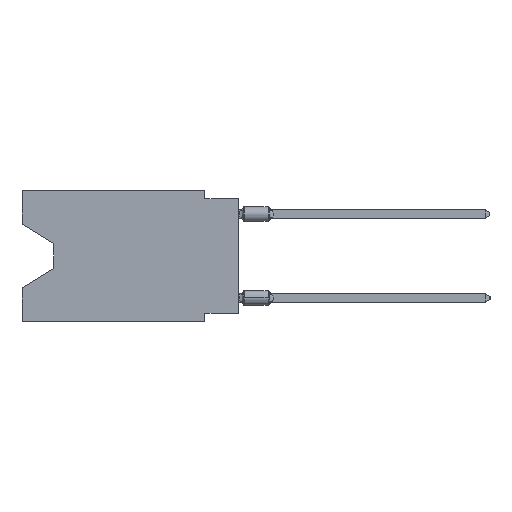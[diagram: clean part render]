
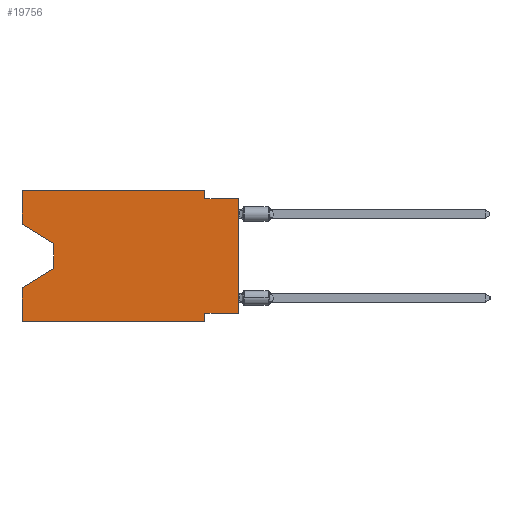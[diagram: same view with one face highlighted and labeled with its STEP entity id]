
A CAD part, left-side view. The second image highlights one B-rep face of the part: STEP entity #19756.
In plain terms, the highlighted planar face has unit normal (-1, 0, 0).
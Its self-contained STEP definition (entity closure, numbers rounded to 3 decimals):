
#735 = EDGE_CURVE ( 'NONE', #19080, #23410, #14116, .T. ) ;
#750 = EDGE_CURVE ( 'NONE', #18447, #24521, #22341, .T. ) ;
#1226 = VERTEX_POINT ( 'NONE', #35129 ) ;
#1673 = CARTESIAN_POINT ( 'NONE',  ( 0., 2.54, -9.906 ) ) ;
#1830 = ORIENTED_EDGE ( 'NONE', *, *, #34242, .T. ) ;
#2940 = LINE ( 'NONE', #16898, #18872 ) ;
#3154 = CARTESIAN_POINT ( 'NONE',  ( 0., 0., 0. ) ) ;
#3334 = VERTEX_POINT ( 'NONE', #30031 ) ;
#3499 = DIRECTION ( 'NONE',  ( 0., 0., 1. ) ) ;
#3804 = VECTOR ( 'NONE', #29965, 1000. ) ;
#3872 = EDGE_CURVE ( 'NONE', #23806, #32056, #2940, .T. ) ;
#4715 = VECTOR ( 'NONE', #9165, 1000. ) ;
#5166 = DIRECTION ( 'NONE',  ( 1., 0., 0. ) ) ;
#5178 = LINE ( 'NONE', #22177, #27597 ) ;
#5519 = VECTOR ( 'NONE', #27559, 1000. ) ;
#5524 = PLANE ( 'NONE',  #31089 ) ;
#5716 = CARTESIAN_POINT ( 'NONE',  ( 0., 13.97, -5.893 ) ) ;
#5723 = LINE ( 'NONE', #16637, #5519 ) ;
#6647 = CARTESIAN_POINT ( 'NONE',  ( 0., 16.383, 0. ) ) ;
#7256 = VERTEX_POINT ( 'NONE', #1673 ) ;
#7344 = ORIENTED_EDGE ( 'NONE', *, *, #23387, .T. ) ;
#7484 = DIRECTION ( 'NONE',  ( 0., 0., 1. ) ) ;
#7715 = ORIENTED_EDGE ( 'NONE', *, *, #8656, .T. ) ;
#8090 = ORIENTED_EDGE ( 'NONE', *, *, #29186, .F. ) ;
#8298 = LINE ( 'NONE', #16544, #3804 ) ;
#8651 = DIRECTION ( 'NONE',  ( 0., 0.855, -0.519 ) ) ;
#8656 = EDGE_CURVE ( 'NONE', #31362, #3334, #27870, .T. ) ;
#9117 = VECTOR ( 'NONE', #14319, 1000. ) ;
#9165 = DIRECTION ( 'NONE',  ( 0., 0., -1. ) ) ;
#9995 = ORIENTED_EDGE ( 'NONE', *, *, #19413, .F. ) ;
#10466 = LINE ( 'NONE', #21583, #16345 ) ;
#11250 = FACE_OUTER_BOUND ( 'NONE', #31777, .T. ) ;
#11430 = DIRECTION ( 'NONE',  ( 0., -1., 0. ) ) ;
#12845 = CARTESIAN_POINT ( 'NONE',  ( 0., 16.383, 0. ) ) ;
#13225 = LINE ( 'NONE', #26847, #4715 ) ;
#13227 = VECTOR ( 'NONE', #33432, 1000. ) ;
#13582 = CARTESIAN_POINT ( 'NONE',  ( 0., 16.383, 0. ) ) ;
#13848 = EDGE_CURVE ( 'NONE', #23806, #7256, #8298, .T. ) ;
#14116 = LINE ( 'NONE', #30246, #22377 ) ;
#14216 = VERTEX_POINT ( 'NONE', #5716 ) ;
#14256 = ORIENTED_EDGE ( 'NONE', *, *, #34443, .F. ) ;
#14319 = DIRECTION ( 'NONE',  ( 0., 0., -1. ) ) ;
#15009 = CARTESIAN_POINT ( 'NONE',  ( 0., 2.54, -9.906 ) ) ;
#15659 = ORIENTED_EDGE ( 'NONE', *, *, #3872, .F. ) ;
#15856 = DIRECTION ( 'NONE',  ( 0., 1., 0. ) ) ;
#16086 = DIRECTION ( 'NONE',  ( 0., 0., -1. ) ) ;
#16345 = VECTOR ( 'NONE', #15856, 1000. ) ;
#16544 = CARTESIAN_POINT ( 'NONE',  ( 0., 16.383, -9.906 ) ) ;
#16637 = CARTESIAN_POINT ( 'NONE',  ( 0., 0., -0.635 ) ) ;
#16898 = CARTESIAN_POINT ( 'NONE',  ( 0., 16.383, 0. ) ) ;
#18447 = VERTEX_POINT ( 'NONE', #23692 ) ;
#18872 = VECTOR ( 'NONE', #19949, 1000. ) ;
#19080 = VERTEX_POINT ( 'NONE', #6647 ) ;
#19363 = VECTOR ( 'NONE', #3499, 1000. ) ;
#19413 = EDGE_CURVE ( 'NONE', #1226, #7256, #30805, .T. ) ;
#19756 = ADVANCED_FACE ( 'NONE', ( #11250 ), #5524, .F. ) ;
#19949 = DIRECTION ( 'NONE',  ( 0., 0., 1. ) ) ;
#21260 = EDGE_CURVE ( 'NONE', #18447, #19080, #31859, .T. ) ;
#21583 = CARTESIAN_POINT ( 'NONE',  ( 0., 0., -9.271 ) ) ;
#22177 = CARTESIAN_POINT ( 'NONE',  ( 0., 2.54, 0. ) ) ;
#22341 = LINE ( 'NONE', #33258, #13227 ) ;
#22377 = VECTOR ( 'NONE', #11430, 1000. ) ;
#22572 = VECTOR ( 'NONE', #7484, 1000. ) ;
#22596 = CARTESIAN_POINT ( 'NONE',  ( 0., 2.54, 0. ) ) ;
#22776 = CARTESIAN_POINT ( 'NONE',  ( 0., 13.97, -5.893 ) ) ;
#22939 = LINE ( 'NONE', #22776, #24885 ) ;
#23387 = EDGE_CURVE ( 'NONE', #14216, #32056, #22939, .T. ) ;
#23410 = VERTEX_POINT ( 'NONE', #22596 ) ;
#23692 = CARTESIAN_POINT ( 'NONE',  ( 0., 16.383, -2.546 ) ) ;
#23806 = VERTEX_POINT ( 'NONE', #27946 ) ;
#24521 = VERTEX_POINT ( 'NONE', #29061 ) ;
#24885 = VECTOR ( 'NONE', #8651, 1000. ) ;
#25238 = ORIENTED_EDGE ( 'NONE', *, *, #750, .T. ) ;
#26473 = ORIENTED_EDGE ( 'NONE', *, *, #21260, .F. ) ;
#26847 = CARTESIAN_POINT ( 'NONE',  ( 0., 13.97, -4.013 ) ) ;
#27559 = DIRECTION ( 'NONE',  ( 0., -1., 0. ) ) ;
#27597 = VECTOR ( 'NONE', #29714, 1000. ) ;
#27870 = LINE ( 'NONE', #3154, #19363 ) ;
#27946 = CARTESIAN_POINT ( 'NONE',  ( 0., 16.383, -9.906 ) ) ;
#28513 = VERTEX_POINT ( 'NONE', #31434 ) ;
#28740 = ORIENTED_EDGE ( 'NONE', *, *, #13848, .T. ) ;
#29061 = CARTESIAN_POINT ( 'NONE',  ( 0., 13.97, -4.013 ) ) ;
#29186 = EDGE_CURVE ( 'NONE', #28513, #3334, #5723, .T. ) ;
#29714 = DIRECTION ( 'NONE',  ( 0., 0., -1. ) ) ;
#29905 = EDGE_CURVE ( 'NONE', #31362, #1226, #10466, .T. ) ;
#29965 = DIRECTION ( 'NONE',  ( 0., -1., 0. ) ) ;
#30031 = CARTESIAN_POINT ( 'NONE',  ( 0., 0., -0.635 ) ) ;
#30246 = CARTESIAN_POINT ( 'NONE',  ( 0., 16.383, 0. ) ) ;
#30801 = CARTESIAN_POINT ( 'NONE',  ( 0., 16.383, -7.36 ) ) ;
#30805 = LINE ( 'NONE', #15009, #9117 ) ;
#31089 = AXIS2_PLACEMENT_3D ( 'NONE', #13582, #5166, #16086 ) ;
#31362 = VERTEX_POINT ( 'NONE', #31568 ) ;
#31434 = CARTESIAN_POINT ( 'NONE',  ( 0., 2.54, -0.635 ) ) ;
#31568 = CARTESIAN_POINT ( 'NONE',  ( 0., 0., -9.271 ) ) ;
#31777 = EDGE_LOOP ( 'NONE', ( #25238, #1830, #7344, #15659, #28740, #9995, #32525, #7715, #8090, #14256, #35142, #26473 ) ) ;
#31859 = LINE ( 'NONE', #12845, #22572 ) ;
#32056 = VERTEX_POINT ( 'NONE', #30801 ) ;
#32525 = ORIENTED_EDGE ( 'NONE', *, *, #29905, .F. ) ;
#33258 = CARTESIAN_POINT ( 'NONE',  ( 0., 16.383, -2.546 ) ) ;
#33432 = DIRECTION ( 'NONE',  ( 0., -0.855, -0.519 ) ) ;
#34242 = EDGE_CURVE ( 'NONE', #24521, #14216, #13225, .T. ) ;
#34443 = EDGE_CURVE ( 'NONE', #23410, #28513, #5178, .T. ) ;
#35129 = CARTESIAN_POINT ( 'NONE',  ( 0., 2.54, -9.271 ) ) ;
#35142 = ORIENTED_EDGE ( 'NONE', *, *, #735, .F. ) ;
